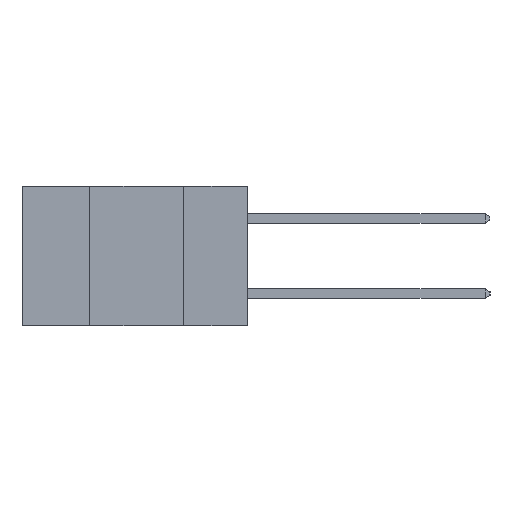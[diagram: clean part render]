
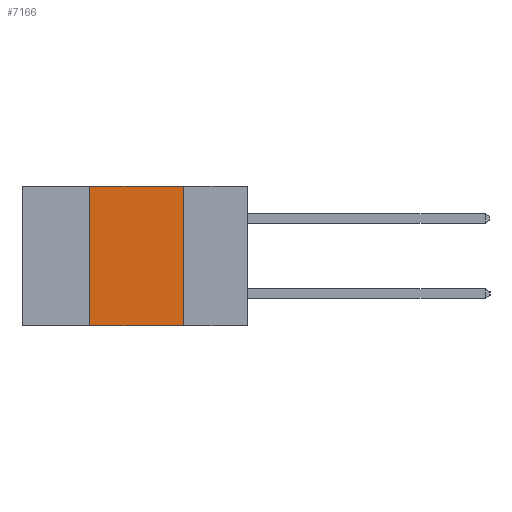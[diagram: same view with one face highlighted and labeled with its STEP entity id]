
A CAD part, left-side view. The second image highlights one B-rep face of the part: STEP entity #7166.
In plain terms, the highlighted planar face has unit normal (-1, 0, 0).
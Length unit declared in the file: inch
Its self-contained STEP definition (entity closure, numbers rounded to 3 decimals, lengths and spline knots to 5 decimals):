
#401 = EDGE_CURVE ( 'NONE', #6184, #7692, #9035, .T. ) ;
#655 = DIRECTION ( 'NONE',  ( 1., 0., 0. ) ) ;
#1077 = ORIENTED_EDGE ( 'NONE', *, *, #4392, .T. ) ;
#1167 = VECTOR ( 'NONE', #6601, 39.37008 ) ;
#1246 = EDGE_LOOP ( 'NONE', ( #1322, #1460, #1503, #1077 ) ) ;
#1322 = ORIENTED_EDGE ( 'NONE', *, *, #8524, .F. ) ;
#1460 = ORIENTED_EDGE ( 'NONE', *, *, #401, .F. ) ;
#1503 = ORIENTED_EDGE ( 'NONE', *, *, #6402, .F. ) ;
#1579 = VERTEX_POINT ( 'NONE', #4896 ) ;
#2237 = CARTESIAN_POINT ( 'NONE',  ( 0., 0.17, 0. ) ) ;
#3175 = VECTOR ( 'NONE', #4181, 39.37008 ) ;
#3358 = LINE ( 'NONE', #6990, #1167 ) ;
#3641 = CARTESIAN_POINT ( 'NONE',  ( 0., 0.42, 0. ) ) ;
#3801 = CARTESIAN_POINT ( 'NONE',  ( 0., 0.17, -0.37 ) ) ;
#4102 = CARTESIAN_POINT ( 'NONE',  ( 0., 0.6, 0. ) ) ;
#4181 = DIRECTION ( 'NONE',  ( 0., -1., 0. ) ) ;
#4392 = EDGE_CURVE ( 'NONE', #1579, #8064, #3358, .T. ) ;
#4895 = DIRECTION ( 'NONE',  ( 0., 0., -1. ) ) ;
#4896 = CARTESIAN_POINT ( 'NONE',  ( 0., 0.42, -0.37 ) ) ;
#5205 = AXIS2_PLACEMENT_3D ( 'NONE', #5472, #655, #6230 ) ;
#5255 = VECTOR ( 'NONE', #9851, 39.37008 ) ;
#5472 = CARTESIAN_POINT ( 'NONE',  ( 0., 0.6, 0. ) ) ;
#6184 = VERTEX_POINT ( 'NONE', #3641 ) ;
#6230 = DIRECTION ( 'NONE',  ( 0., 0., -1. ) ) ;
#6402 = EDGE_CURVE ( 'NONE', #1579, #6184, #7445, .T. ) ;
#6583 = CARTESIAN_POINT ( 'NONE',  ( 0., 0.17, -0.37 ) ) ;
#6601 = DIRECTION ( 'NONE',  ( 0., -1., 0. ) ) ;
#6990 = CARTESIAN_POINT ( 'NONE',  ( 0., 0.6, -0.37 ) ) ;
#7166 = ADVANCED_FACE ( 'NONE', ( #8508 ), #9729, .F. ) ;
#7445 = LINE ( 'NONE', #9591, #5255 ) ;
#7692 = VERTEX_POINT ( 'NONE', #2237 ) ;
#8064 = VERTEX_POINT ( 'NONE', #6583 ) ;
#8508 = FACE_OUTER_BOUND ( 'NONE', #1246, .T. ) ;
#8524 = EDGE_CURVE ( 'NONE', #7692, #8064, #9568, .T. ) ;
#9035 = LINE ( 'NONE', #4102, #3175 ) ;
#9351 = VECTOR ( 'NONE', #4895, 39.37008 ) ;
#9568 = LINE ( 'NONE', #3801, #9351 ) ;
#9591 = CARTESIAN_POINT ( 'NONE',  ( 0., 0.42, -0.37 ) ) ;
#9729 = PLANE ( 'NONE',  #5205 ) ;
#9851 = DIRECTION ( 'NONE',  ( 0., 0., 1. ) ) ;
